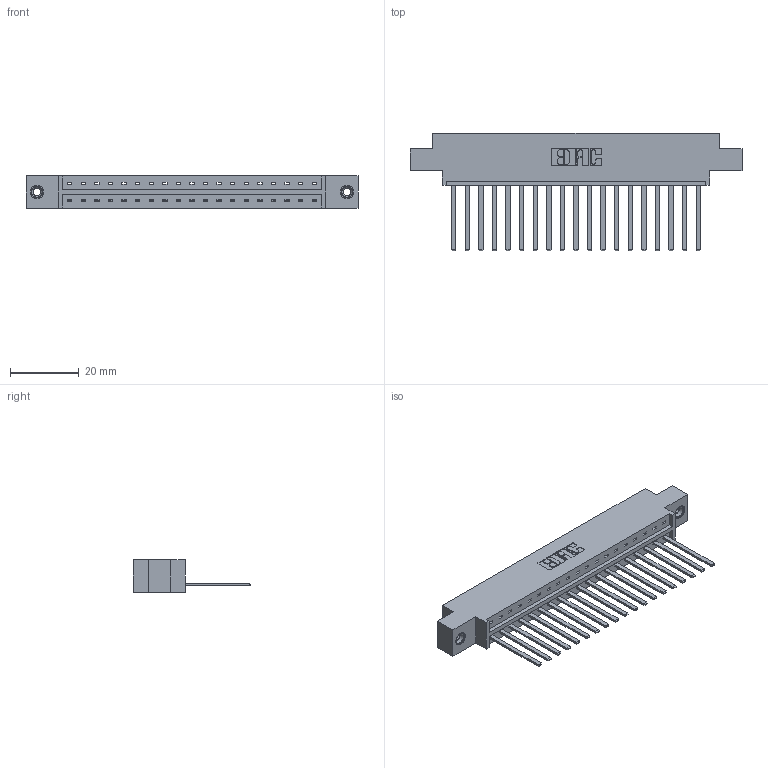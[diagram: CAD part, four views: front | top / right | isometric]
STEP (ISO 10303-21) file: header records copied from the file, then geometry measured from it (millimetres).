
FILE_DESCRIPTION (( 'STEP AP203' ), '1' );
FILE_NAME ('833-019-544-608.STEP', '2020-06-01T00:51:43', ( '' ), ( '' ), 'SwSTEP 2.0', 'SolidWorks 2020', '' );
FILE_SCHEMA (( 'CONFIG_CONTROL_DESIGN' ));
Length unit declared in the file: inch
Products named in the file (4): 345-250-001_345-250-003-102; 345-292-001_345-293-144; 833 Part_Offset - .156 Dia - TI; 833-019-544-608
Assembly tree (22 placements, depth 2):
  833-019-544-608
    833 Part_Offset - .156 Dia - TI
    345-292-001_345-293-144  x19
    345-250-001_345-250-003-102  x2
Bounding box: 96.82 x 34.3 x 9.4 mm (x, y, z)
Volume: 9531.2 mm3; surface area: 11101.4 mm2
Topology: 22 solids, 22 shells, 1166 faces, 3461 edges, 2274 vertices
Faces by surface type: plane 828, cylinder 322, cone 12, torus 4
Entity records: 15724 total; most frequent: CARTESIAN_POINT 2698, ORIENTED_EDGE 2646, DIRECTION 2351, EDGE_CURVE 1323, VECTOR 1179, LINE 1179, VERTEX_POINT 876, AXIS2_PLACEMENT_3D 586
